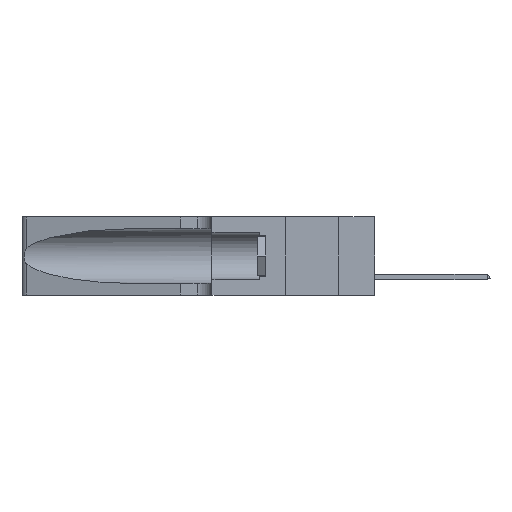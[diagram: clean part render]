
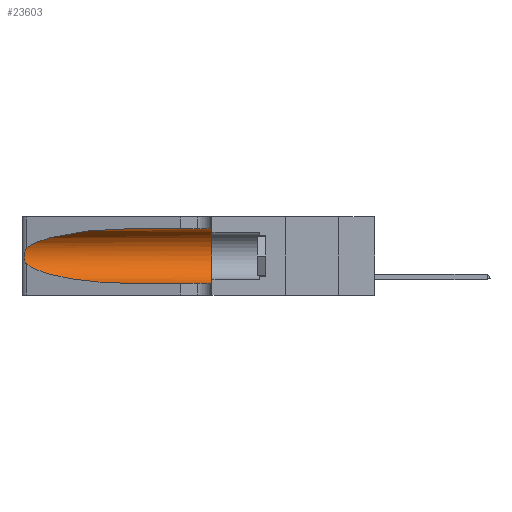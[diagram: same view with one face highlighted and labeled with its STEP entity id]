
A CAD part, left-side view. The second image highlights one B-rep face of the part: STEP entity #23603.
In plain terms, the highlighted cylindrical face has radius 3.308 mm (diameter 6.617 mm), a partial arc.
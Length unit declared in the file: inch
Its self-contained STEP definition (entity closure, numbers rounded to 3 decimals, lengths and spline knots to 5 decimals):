
#271 = B_SPLINE_CURVE_WITH_KNOTS ( 'NONE', 3,
 ( #16630, #24255, #20224, #7966, #22302, #18400, #8487, #14757, #22834, #2504, #4362, #14851, #2323, #14583 ),
 .UNSPECIFIED., .F., .F.,
 ( 4, 2, 2, 2, 2, 2, 4 ),
 ( 0., 0.00027, 0.00053, 0.00107, 0.0016, 0.00187, 0.00214 ),
 .UNSPECIFIED. ) ;
#635 = EDGE_CURVE ( 'NONE', #23420, #7351, #12485, .T. ) ;
#750 = DIRECTION ( 'NONE',  ( 0., -1., 0. ) ) ;
#1081 = CARTESIAN_POINT ( 'NONE',  ( 0.25487, 1.22718, 0.22369 ) ) ;
#1433 =( BOUNDED_CURVE ( )  B_SPLINE_CURVE ( 3, ( #6101, #3808, #8179, #22263 ),
 .UNSPECIFIED., .F., .F. ) 
 B_SPLINE_CURVE_WITH_KNOTS ( ( 4, 4 ),
 ( 3.44316, 4.71239 ),
 .UNSPECIFIED. ) 
 CURVE ( )  GEOMETRIC_REPRESENTATION_ITEM ( )  RATIONAL_B_SPLINE_CURVE ( ( 1., 0.87, 0.87, 1. ) ) 
 REPRESENTATION_ITEM ( '' )  );
#2003 = CARTESIAN_POINT ( 'NONE',  ( 0.1305, 0.72297, 0.31525 ) ) ;
#2323 = CARTESIAN_POINT ( 'NONE',  ( 0.25555, 1.22993, 0.14849 ) ) ;
#2504 = CARTESIAN_POINT ( 'NONE',  ( 0.25856, 1.23593, 0.16098 ) ) ;
#2671 = EDGE_CURVE ( 'NONE', #4184, #23420, #1433, .T. ) ;
#3119 = ORIENTED_EDGE ( 'NONE', *, *, #635, .T. ) ;
#3129 = VERTEX_POINT ( 'NONE', #2003 ) ;
#3764 = ORIENTED_EDGE ( 'NONE', *, *, #7389, .T. ) ;
#3808 = CARTESIAN_POINT ( 'NONE',  ( 0.2373, 1.15595, 0.08982 ) ) ;
#4184 = VERTEX_POINT ( 'NONE', #23231 ) ;
#4362 = CARTESIAN_POINT ( 'NONE',  ( 0.25789, 1.23486, 0.15765 ) ) ;
#4678 = CARTESIAN_POINT ( 'NONE',  ( 0.1305, 1.61858, 0.185 ) ) ;
#4915 = DIRECTION ( 'NONE',  ( 0., -1., 0. ) ) ;
#5363 = CARTESIAN_POINT ( 'NONE',  ( 0.1305, 0.72297, 0.31525 ) ) ;
#5448 = CARTESIAN_POINT ( 'NONE',  ( 0.2373, 1.15595, 0.28018 ) ) ;
#6101 = CARTESIAN_POINT ( 'NONE',  ( 0.25487, 1.22718, 0.14631 ) ) ;
#6696 = VERTEX_POINT ( 'NONE', #1081 ) ;
#7351 = VERTEX_POINT ( 'NONE', #23822 ) ;
#7376 = CARTESIAN_POINT ( 'NONE',  ( 0.1305, 0.35, 0.31525 ) ) ;
#7389 = EDGE_CURVE ( 'NONE', #3129, #6696, #19304, .T. ) ;
#7598 = CARTESIAN_POINT ( 'NONE',  ( 0.18966, 0.96281, 0.31525 ) ) ;
#7966 = CARTESIAN_POINT ( 'NONE',  ( 0.25787, 1.23484, 0.2124 ) ) ;
#8179 = CARTESIAN_POINT ( 'NONE',  ( 0.18966, 0.96281, 0.05475 ) ) ;
#8487 = CARTESIAN_POINT ( 'NONE',  ( 0.26075, 1.23896, 0.19203 ) ) ;
#9930 = EDGE_CURVE ( 'NONE', #10610, #7351, #25250, .T. ) ;
#10610 = VERTEX_POINT ( 'NONE', #7376 ) ;
#11382 = CARTESIAN_POINT ( 'NONE',  ( 0.25487, 1.22718, 0.22369 ) ) ;
#12243 = CARTESIAN_POINT ( 'NONE',  ( 0.1305, 0.35, 0.185 ) ) ;
#12485 = LINE ( 'NONE', #25327, #15350 ) ;
#12606 = DIRECTION ( 'NONE',  ( 0., 0., 1. ) ) ;
#13131 = DIRECTION ( 'NONE',  ( 0., 0., -1. ) ) ;
#14583 = CARTESIAN_POINT ( 'NONE',  ( 0.25487, 1.22718, 0.14631 ) ) ;
#14757 = CARTESIAN_POINT ( 'NONE',  ( 0.26075, 1.23896, 0.178 ) ) ;
#14851 = CARTESIAN_POINT ( 'NONE',  ( 0.25639, 1.23186, 0.15144 ) ) ;
#15350 = VECTOR ( 'NONE', #4915, 39.37008 ) ;
#15713 = EDGE_CURVE ( 'NONE', #6696, #4184, #271, .T. ) ;
#16017 = AXIS2_PLACEMENT_3D ( 'NONE', #4678, #17011, #13131 ) ;
#16416 = AXIS2_PLACEMENT_3D ( 'NONE', #12243, #24824, #12606 ) ;
#16630 = CARTESIAN_POINT ( 'NONE',  ( 0.25487, 1.22718, 0.22369 ) ) ;
#16738 = ORIENTED_EDGE ( 'NONE', *, *, #15713, .T. ) ;
#17011 = DIRECTION ( 'NONE',  ( 0., -1., 0. ) ) ;
#17362 = CARTESIAN_POINT ( 'NONE',  ( 0.1305, 1.61858, 0.31525 ) ) ;
#17637 = ORIENTED_EDGE ( 'NONE', *, *, #9930, .F. ) ;
#18400 = CARTESIAN_POINT ( 'NONE',  ( 0.26018, 1.23835, 0.19895 ) ) ;
#19304 =( BOUNDED_CURVE ( )  B_SPLINE_CURVE ( 3, ( #5363, #7598, #5448, #11382 ),
 .UNSPECIFIED., .F., .T. ) 
 B_SPLINE_CURVE_WITH_KNOTS ( ( 4, 4 ),
 ( 1.5708, 2.84003 ),
 .UNSPECIFIED. ) 
 CURVE ( )  GEOMETRIC_REPRESENTATION_ITEM ( )  RATIONAL_B_SPLINE_CURVE ( ( 1., 0.87, 0.87, 1. ) ) 
 REPRESENTATION_ITEM ( '' )  );
#20128 = CARTESIAN_POINT ( 'NONE',  ( 0.1305, 0.72297, 0.05475 ) ) ;
#20224 = CARTESIAN_POINT ( 'NONE',  ( 0.25639, 1.23184, 0.21858 ) ) ;
#21301 = ORIENTED_EDGE ( 'NONE', *, *, #25545, .F. ) ;
#21679 = ORIENTED_EDGE ( 'NONE', *, *, #2671, .T. ) ;
#22263 = CARTESIAN_POINT ( 'NONE',  ( 0.1305, 0.72297, 0.05475 ) ) ;
#22302 = CARTESIAN_POINT ( 'NONE',  ( 0.25854, 1.2359, 0.20912 ) ) ;
#22783 = LINE ( 'NONE', #17362, #24350 ) ;
#22834 = CARTESIAN_POINT ( 'NONE',  ( 0.26017, 1.23833, 0.17102 ) ) ;
#23231 = CARTESIAN_POINT ( 'NONE',  ( 0.25487, 1.22718, 0.14631 ) ) ;
#23420 = VERTEX_POINT ( 'NONE', #20128 ) ;
#23603 = ADVANCED_FACE ( 'NONE', ( #25129 ), #24478, .F. ) ;
#23822 = CARTESIAN_POINT ( 'NONE',  ( 0.1305, 0.35, 0.05475 ) ) ;
#24255 = CARTESIAN_POINT ( 'NONE',  ( 0.25555, 1.22994, 0.2215 ) ) ;
#24350 = VECTOR ( 'NONE', #750, 39.37008 ) ;
#24478 = CYLINDRICAL_SURFACE ( 'NONE', #16017, 0.13025 ) ;
#24824 = DIRECTION ( 'NONE',  ( 0., 1., 0. ) ) ;
#25129 = FACE_OUTER_BOUND ( 'NONE', #25451, .T. ) ;
#25250 = CIRCLE ( 'NONE', #16416, 0.13025 ) ;
#25327 = CARTESIAN_POINT ( 'NONE',  ( 0.1305, 1.61858, 0.05475 ) ) ;
#25451 = EDGE_LOOP ( 'NONE', ( #3764, #16738, #21679, #3119, #17637, #21301 ) ) ;
#25545 = EDGE_CURVE ( 'NONE', #3129, #10610, #22783, .T. ) ;
